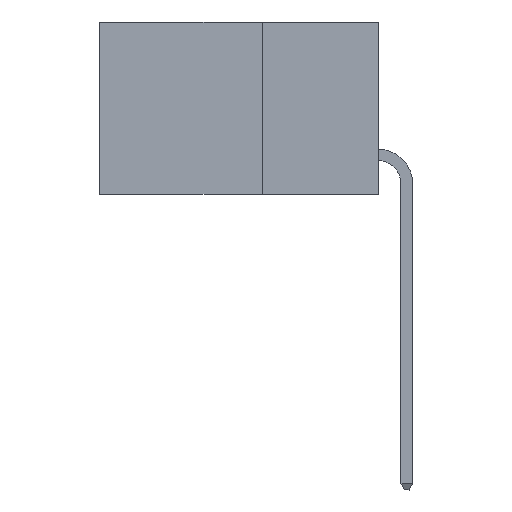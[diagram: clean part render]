
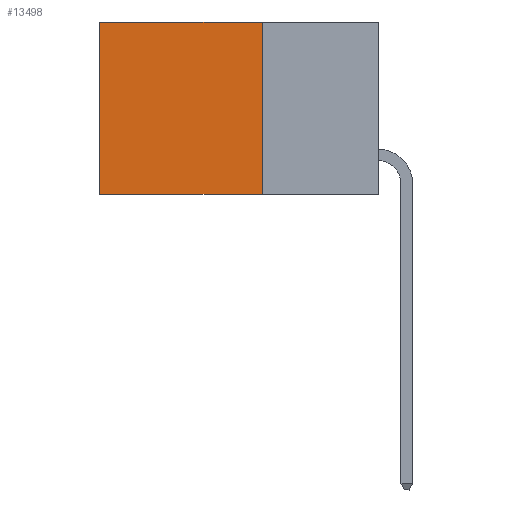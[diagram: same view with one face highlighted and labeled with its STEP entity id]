
A CAD part, left-side view. The second image highlights one B-rep face of the part: STEP entity #13498.
In plain terms, the highlighted planar face has unit normal (-1, 0, 0).
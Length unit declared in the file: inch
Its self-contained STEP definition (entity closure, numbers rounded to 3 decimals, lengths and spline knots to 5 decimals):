
#139 = VERTEX_POINT ( 'NONE', #11537 ) ;
#689 = CARTESIAN_POINT ( 'NONE',  ( 0.298, 0.25, -0.37 ) ) ;
#1007 = CARTESIAN_POINT ( 'NONE',  ( 0.298, 0.6, 0. ) ) ;
#1822 = EDGE_CURVE ( 'NONE', #12129, #12763, #19535, .T. ) ;
#2415 = LINE ( 'NONE', #4438, #18061 ) ;
#2988 = ORIENTED_EDGE ( 'NONE', *, *, #17530, .T. ) ;
#4021 = CARTESIAN_POINT ( 'NONE',  ( 0.298, 0.25, 0. ) ) ;
#4438 = CARTESIAN_POINT ( 'NONE',  ( 0.298, 0.25, 0. ) ) ;
#5380 = VECTOR ( 'NONE', #5594, 39.37008 ) ;
#5594 = DIRECTION ( 'NONE',  ( 0., 0., -1. ) ) ;
#5744 = DIRECTION ( 'NONE',  ( 0., 0., -1. ) ) ;
#6780 = PLANE ( 'NONE',  #19539 ) ;
#7003 = ORIENTED_EDGE ( 'NONE', *, *, #1822, .F. ) ;
#8324 = DIRECTION ( 'NONE',  ( 0., 0., -1. ) ) ;
#8764 = LINE ( 'NONE', #1007, #12485 ) ;
#9281 = FACE_OUTER_BOUND ( 'NONE', #10987, .T. ) ;
#9785 = DIRECTION ( 'NONE',  ( 0., 1., 0. ) ) ;
#10720 = VECTOR ( 'NONE', #9785, 39.37008 ) ;
#10813 = CARTESIAN_POINT ( 'NONE',  ( 0.298, 0.25, -0.37 ) ) ;
#10987 = EDGE_LOOP ( 'NONE', ( #2988, #7003, #16398, #20079 ) ) ;
#11002 = CARTESIAN_POINT ( 'NONE',  ( 0.298, 0.6, 0. ) ) ;
#11419 = CARTESIAN_POINT ( 'NONE',  ( 0.298, 0.25, 0. ) ) ;
#11537 = CARTESIAN_POINT ( 'NONE',  ( 0.298, 0.25, 0. ) ) ;
#11715 = EDGE_CURVE ( 'NONE', #139, #15521, #2415, .T. ) ;
#12129 = VERTEX_POINT ( 'NONE', #689 ) ;
#12485 = VECTOR ( 'NONE', #5744, 39.37008 ) ;
#12763 = VERTEX_POINT ( 'NONE', #17799 ) ;
#13498 = ADVANCED_FACE ( 'NONE', ( #9281 ), #6780, .F. ) ;
#13704 = LINE ( 'NONE', #4021, #5380 ) ;
#15467 = DIRECTION ( 'NONE',  ( 0., 1., 0. ) ) ;
#15521 = VERTEX_POINT ( 'NONE', #11002 ) ;
#16398 = ORIENTED_EDGE ( 'NONE', *, *, #18092, .F. ) ;
#17530 = EDGE_CURVE ( 'NONE', #15521, #12763, #8764, .T. ) ;
#17751 = DIRECTION ( 'NONE',  ( 1., 0., 0. ) ) ;
#17799 = CARTESIAN_POINT ( 'NONE',  ( 0.298, 0.6, -0.37 ) ) ;
#18061 = VECTOR ( 'NONE', #15467, 39.37008 ) ;
#18092 = EDGE_CURVE ( 'NONE', #139, #12129, #13704, .T. ) ;
#19535 = LINE ( 'NONE', #10813, #10720 ) ;
#19539 = AXIS2_PLACEMENT_3D ( 'NONE', #11419, #17751, #8324 ) ;
#20079 = ORIENTED_EDGE ( 'NONE', *, *, #11715, .T. ) ;
